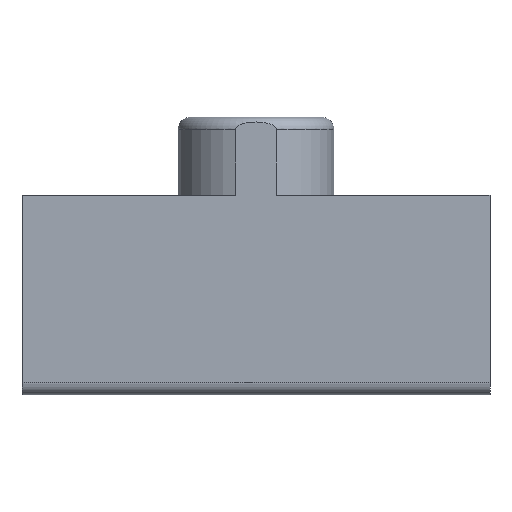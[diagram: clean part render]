
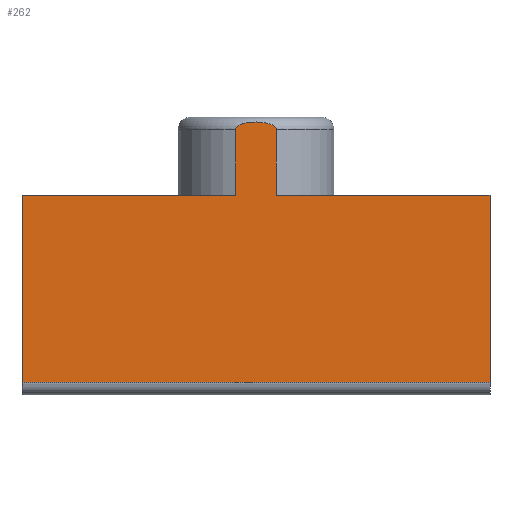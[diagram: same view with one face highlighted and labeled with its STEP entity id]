
A CAD part, left-side view. The second image highlights one B-rep face of the part: STEP entity #262.
In plain terms, the highlighted planar face has unit normal (-1, 0, 0).
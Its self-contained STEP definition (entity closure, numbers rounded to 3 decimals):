
#15=B_SPLINE_CURVE_WITH_KNOTS('',3,(#418,#419,#420,#421,#422,#423,#424,
#425,#426,#427),.UNSPECIFIED.,.F.,.F.,(4,2,2,2,4),(-0.269,-0.263,
-0.254,-0.24,-0.179),.UNSPECIFIED.);
#17=B_SPLINE_CURVE_WITH_KNOTS('',3,(#448,#449,#450,#451,#452,#453,#454,
#455,#456,#457),.UNSPECIFIED.,.F.,.F.,(4,2,2,2,4),(-0.179,-0.119,
-0.104,-0.096,-0.09),
 .UNSPECIFIED.);
#50=FACE_OUTER_BOUND('',#66,.T.);
#66=EDGE_LOOP('',(#229,#230,#231,#232,#233,#234,#235,#236,#237));
#73=LINE('',#402,#94);
#74=LINE('',#406,#95);
#76=LINE('',#460,#97);
#80=LINE('',#472,#101);
#83=LINE('',#478,#104);
#84=LINE('',#480,#105);
#87=LINE('',#485,#108);
#94=VECTOR('',#327,10.);
#95=VECTOR('',#330,10.);
#97=VECTOR('',#346,10.);
#101=VECTOR('',#358,10.);
#104=VECTOR('',#363,10.);
#105=VECTOR('',#366,10.);
#108=VECTOR('',#373,10.);
#117=VERTEX_POINT('',#398);
#118=VERTEX_POINT('',#400);
#119=VERTEX_POINT('',#404);
#120=VERTEX_POINT('',#405);
#124=VERTEX_POINT('',#415);
#125=VERTEX_POINT('',#417);
#127=VERTEX_POINT('',#459);
#131=VERTEX_POINT('',#470);
#133=VERTEX_POINT('',#476);
#144=EDGE_CURVE('',#118,#117,#73,.T.);
#145=EDGE_CURVE('',#119,#120,#74,.T.);
#151=EDGE_CURVE('',#124,#125,#15,.F.);
#154=EDGE_CURVE('',#120,#124,#17,.F.);
#155=EDGE_CURVE('',#125,#127,#76,.T.);
#161=EDGE_CURVE('',#131,#118,#80,.T.);
#164=EDGE_CURVE('',#133,#119,#83,.T.);
#165=EDGE_CURVE('',#127,#131,#84,.T.);
#168=EDGE_CURVE('',#133,#117,#87,.T.);
#229=ORIENTED_EDGE('',*,*,#161,.F.);
#230=ORIENTED_EDGE('',*,*,#165,.F.);
#231=ORIENTED_EDGE('',*,*,#155,.F.);
#232=ORIENTED_EDGE('',*,*,#151,.F.);
#233=ORIENTED_EDGE('',*,*,#154,.F.);
#234=ORIENTED_EDGE('',*,*,#145,.F.);
#235=ORIENTED_EDGE('',*,*,#164,.F.);
#236=ORIENTED_EDGE('',*,*,#168,.T.);
#237=ORIENTED_EDGE('',*,*,#144,.F.);
#249=PLANE('',#302);
#262=ADVANCED_FACE('',(#50),#249,.T.);
#302=AXIS2_PLACEMENT_3D('',#486,#374,#375);
#327=DIRECTION('',(0.,1.,0.));
#330=DIRECTION('',(0.,0.,1.));
#346=DIRECTION('',(0.,0.,-1.));
#358=DIRECTION('',(0.,0.,-1.));
#363=DIRECTION('',(0.,-1.,0.));
#366=DIRECTION('',(0.,-1.,0.));
#373=DIRECTION('',(0.,0.,-1.));
#374=DIRECTION('center_axis',(-1.,0.,0.));
#375=DIRECTION('ref_axis',(0.,1.,0.));
#398=CARTESIAN_POINT('',(-271.73,-32.3,12.613));
#400=CARTESIAN_POINT('',(-271.73,-51.35,12.613));
#402=CARTESIAN_POINT('',(-271.73,-51.35,12.613));
#404=CARTESIAN_POINT('',(-271.73,-40.997,20.225));
#405=CARTESIAN_POINT('',(-271.73,-40.997,22.892));
#406=CARTESIAN_POINT('',(-271.73,-40.997,20.225));
#415=CARTESIAN_POINT('',(-271.73,-41.825,23.208));
#417=CARTESIAN_POINT('',(-271.73,-42.653,22.892));
#418=CARTESIAN_POINT('Ctrl Pts',(-271.73,-42.653,22.892));
#419=CARTESIAN_POINT('Ctrl Pts',(-271.73,-42.653,22.912));
#420=CARTESIAN_POINT('Ctrl Pts',(-271.73,-42.648,22.935));
#421=CARTESIAN_POINT('Ctrl Pts',(-271.73,-42.627,22.978));
#422=CARTESIAN_POINT('Ctrl Pts',(-271.73,-42.606,23.004));
#423=CARTESIAN_POINT('Ctrl Pts',(-271.73,-42.549,23.056));
#424=CARTESIAN_POINT('Ctrl Pts',(-271.73,-42.498,23.085));
#425=CARTESIAN_POINT('Ctrl Pts',(-271.73,-42.268,23.185));
#426=CARTESIAN_POINT('Ctrl Pts',(-271.73,-42.027,23.208));
#427=CARTESIAN_POINT('Ctrl Pts',(-271.73,-41.825,23.208));
#448=CARTESIAN_POINT('Ctrl Pts',(-271.73,-41.825,23.208));
#449=CARTESIAN_POINT('Ctrl Pts',(-271.73,-41.623,23.208));
#450=CARTESIAN_POINT('Ctrl Pts',(-271.73,-41.382,23.185));
#451=CARTESIAN_POINT('Ctrl Pts',(-271.73,-41.152,23.085));
#452=CARTESIAN_POINT('Ctrl Pts',(-271.73,-41.101,23.056));
#453=CARTESIAN_POINT('Ctrl Pts',(-271.73,-41.044,23.004));
#454=CARTESIAN_POINT('Ctrl Pts',(-271.73,-41.023,22.978));
#455=CARTESIAN_POINT('Ctrl Pts',(-271.73,-41.002,22.935));
#456=CARTESIAN_POINT('Ctrl Pts',(-271.73,-40.997,22.912));
#457=CARTESIAN_POINT('Ctrl Pts',(-271.73,-40.997,22.892));
#459=CARTESIAN_POINT('',(-271.73,-42.653,20.225));
#460=CARTESIAN_POINT('',(-271.73,-42.653,20.225));
#470=CARTESIAN_POINT('',(-271.73,-51.35,20.225));
#472=CARTESIAN_POINT('',(-271.73,-51.35,13.613));
#476=CARTESIAN_POINT('',(-271.73,-32.3,20.225));
#478=CARTESIAN_POINT('',(-271.73,-32.3,20.225));
#480=CARTESIAN_POINT('',(-271.73,-32.3,20.225));
#485=CARTESIAN_POINT('',(-271.73,-32.3,12.736));
#486=CARTESIAN_POINT('Origin',(-271.73,-51.35,20.225));
